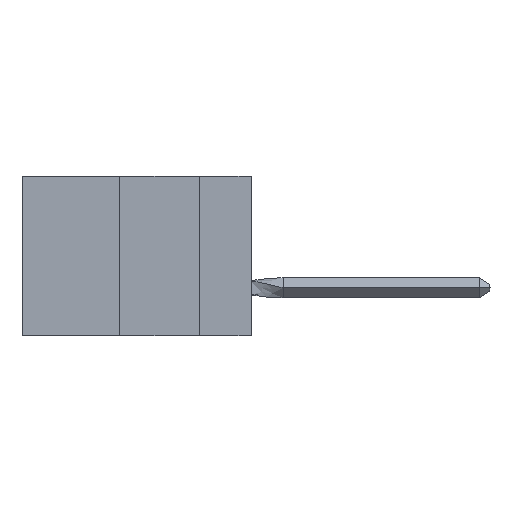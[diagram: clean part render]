
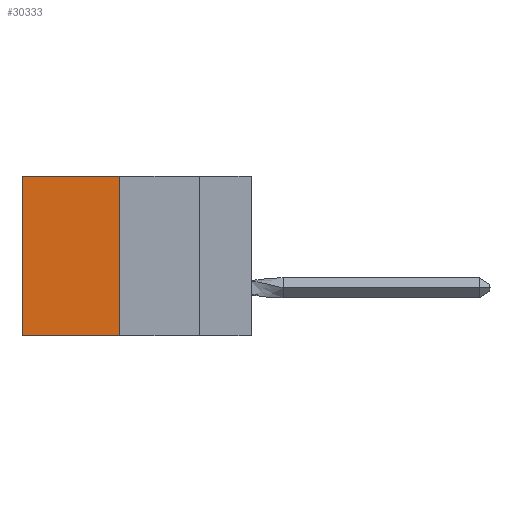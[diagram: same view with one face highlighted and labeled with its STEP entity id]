
A CAD part, left-side view. The second image highlights one B-rep face of the part: STEP entity #30333.
In plain terms, the highlighted planar face has unit normal (-1, 0, 0).
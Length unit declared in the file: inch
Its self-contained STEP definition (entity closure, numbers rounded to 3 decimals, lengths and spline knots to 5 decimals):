
#677 = VERTEX_POINT ( 'NONE', #28647 ) ;
#930 = AXIS2_PLACEMENT_3D ( 'NONE', #10698, #22774, #22277 ) ;
#1694 = CARTESIAN_POINT ( 'NONE',  ( 0.305, 0.413, -0.5 ) ) ;
#3044 = DIRECTION ( 'NONE',  ( 0., 1., 0. ) ) ;
#4247 = VERTEX_POINT ( 'NONE', #19933 ) ;
#7938 = VERTEX_POINT ( 'NONE', #1694 ) ;
#8639 = CARTESIAN_POINT ( 'NONE',  ( 0.305, 0.413, -0.5 ) ) ;
#9379 = LINE ( 'NONE', #8639, #37677 ) ;
#10623 = DIRECTION ( 'NONE',  ( 0., 0., -1. ) ) ;
#10698 = CARTESIAN_POINT ( 'NONE',  ( 0.305, 0.413, -0.5 ) ) ;
#11445 = ORIENTED_EDGE ( 'NONE', *, *, #18215, .F. ) ;
#11517 = EDGE_LOOP ( 'NONE', ( #28982, #13862, #11445, #25376 ) ) ;
#11675 = FACE_OUTER_BOUND ( 'NONE', #11517, .T. ) ;
#13734 = LINE ( 'NONE', #30384, #31979 ) ;
#13862 = ORIENTED_EDGE ( 'NONE', *, *, #22798, .F. ) ;
#13886 = CARTESIAN_POINT ( 'NONE',  ( 0.305, 0.413, 0. ) ) ;
#14848 = CARTESIAN_POINT ( 'NONE',  ( 0.305, 0.413, -0.5 ) ) ;
#18215 = EDGE_CURVE ( 'NONE', #28424, #7938, #27918, .T. ) ;
#18349 = EDGE_CURVE ( 'NONE', #28424, #677, #33047, .T. ) ;
#18540 = CARTESIAN_POINT ( 'NONE',  ( 0.305, 0.413, 0. ) ) ;
#19933 = CARTESIAN_POINT ( 'NONE',  ( 0.305, 0.72, -0.5 ) ) ;
#22277 = DIRECTION ( 'NONE',  ( 0., 0., -1. ) ) ;
#22774 = DIRECTION ( 'NONE',  ( 1., 0., 0. ) ) ;
#22798 = EDGE_CURVE ( 'NONE', #7938, #4247, #9379, .T. ) ;
#25194 = VECTOR ( 'NONE', #33108, 39.37008 ) ;
#25376 = ORIENTED_EDGE ( 'NONE', *, *, #18349, .T. ) ;
#27461 = VECTOR ( 'NONE', #29846, 39.37008 ) ;
#27918 = LINE ( 'NONE', #14848, #27461 ) ;
#28424 = VERTEX_POINT ( 'NONE', #13886 ) ;
#28647 = CARTESIAN_POINT ( 'NONE',  ( 0.305, 0.72, 0. ) ) ;
#28982 = ORIENTED_EDGE ( 'NONE', *, *, #32891, .T. ) ;
#29846 = DIRECTION ( 'NONE',  ( 0., 0., -1. ) ) ;
#30333 = ADVANCED_FACE ( 'NONE', ( #11675 ), #34069, .F. ) ;
#30384 = CARTESIAN_POINT ( 'NONE',  ( 0.305, 0.72, -0.5 ) ) ;
#31979 = VECTOR ( 'NONE', #10623, 39.37008 ) ;
#32891 = EDGE_CURVE ( 'NONE', #677, #4247, #13734, .T. ) ;
#33047 = LINE ( 'NONE', #18540, #25194 ) ;
#33108 = DIRECTION ( 'NONE',  ( 0., 1., 0. ) ) ;
#34069 = PLANE ( 'NONE',  #930 ) ;
#37677 = VECTOR ( 'NONE', #3044, 39.37008 ) ;
